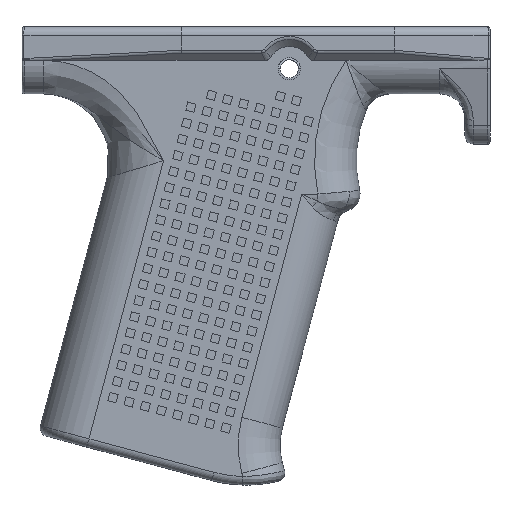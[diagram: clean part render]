
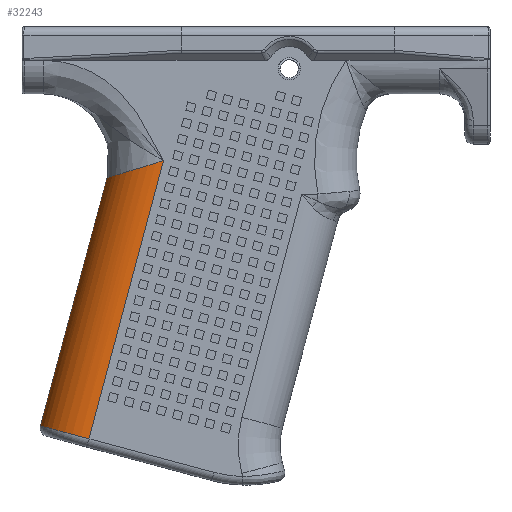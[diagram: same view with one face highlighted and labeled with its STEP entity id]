
A CAD part, top view. The second image highlights one B-rep face of the part: STEP entity #32243.
In plain terms, the highlighted cylindrical face has radius 9.525 mm (diameter 19.05 mm), a partial arc.
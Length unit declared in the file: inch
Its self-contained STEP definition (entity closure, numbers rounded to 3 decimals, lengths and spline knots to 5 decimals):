
#3909=FACE_OUTER_BOUND('',#6047,.T.);
#6047=EDGE_LOOP('',(#30165,#30166,#30167,#30168));
#6207=CIRCLE('',#34172,0.375);
#6381=LINE('',#43279,#10478);
#10317=LINE('',#52034,#14414);
#10478=VECTOR('',#34714,2.15413);
#14414=VECTOR('',#42088,1.91967);
#14484=ELLIPSE('',#34104,0.44226,0.375);
#14659=VERTEX_POINT('',#43258);
#14660=VERTEX_POINT('',#43278);
#17260=VERTEX_POINT('',#51703);
#17296=VERTEX_POINT('',#51966);
#17605=EDGE_CURVE('',#14660,#14659,#6381,.T.);
#21522=EDGE_CURVE('',#17260,#14659,#14484,.T.);
#21593=EDGE_CURVE('',#14660,#17296,#6207,.T.);
#21604=EDGE_CURVE('',#17260,#17296,#10317,.T.);
#30165=ORIENTED_EDGE('',*,*,#21593,.F.);
#30166=ORIENTED_EDGE('',*,*,#17605,.T.);
#30167=ORIENTED_EDGE('',*,*,#21522,.F.);
#30168=ORIENTED_EDGE('',*,*,#21604,.T.);
#30465=CYLINDRICAL_SURFACE('',#34181,0.375);
#32243=ADVANCED_FACE('',(#3909),#30465,.T.);
#34104=AXIS2_PLACEMENT_3D('',#51705,#41904,#41905);
#34172=AXIS2_PLACEMENT_3D('',#52013,#42064,#42065);
#34181=AXIS2_PLACEMENT_3D('',#52036,#42090,#42091);
#34714=DIRECTION('',(0.259,0.966,0.));
#41904=DIRECTION('center_axis',(-0.293,0.956,0.));
#41905=DIRECTION('ref_axis',(-0.956,-0.293,0.));
#42064=DIRECTION('center_axis',(-0.259,-0.966,0.));
#42065=DIRECTION('ref_axis',(-0.683,0.183,0.707));
#42088=DIRECTION('',(-0.259,-0.966,0.));
#42090=DIRECTION('center_axis',(-0.259,-0.966,0.));
#42091=DIRECTION('ref_axis',(-0.683,0.183,0.707));
#43258=CARTESIAN_POINT('',(0.55855,-1.,0.));
#43278=CARTESIAN_POINT('',(0.00102,-3.08073,0.));
#43279=CARTESIAN_POINT('',(0.71882,-0.40184,0.));
#51703=CARTESIAN_POINT('',(0.13564,-1.12941,-0.375));
#51705=CARTESIAN_POINT('Origin',(0.55855,-1.,-0.375));
#51966=CARTESIAN_POINT('',(-0.3612,-2.98367,-0.375));
#52013=CARTESIAN_POINT('Origin',(0.00102,-3.08073,
-0.375));
#52034=CARTESIAN_POINT('',(0.3566,-0.30478,-0.375));
#52036=CARTESIAN_POINT('Origin',(0.71882,-0.40184,-0.375));
